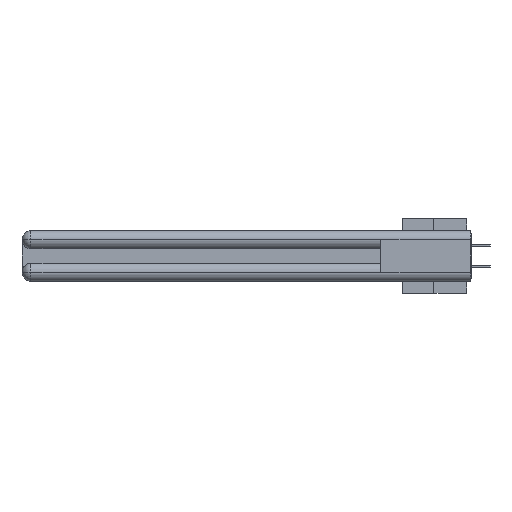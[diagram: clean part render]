
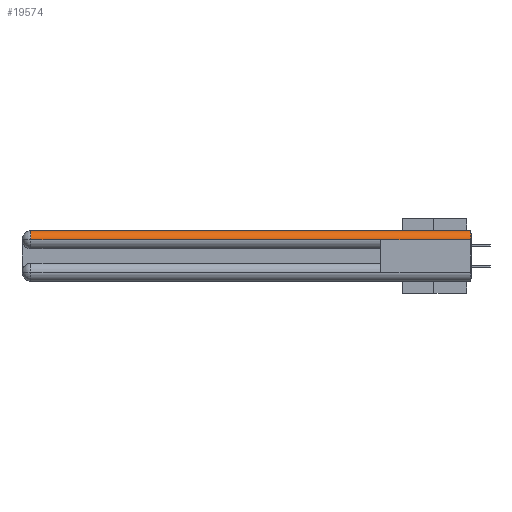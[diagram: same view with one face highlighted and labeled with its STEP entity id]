
A CAD part, left-side view. The second image highlights one B-rep face of the part: STEP entity #19574.
In plain terms, the highlighted cylindrical face has radius 1.562 mm (diameter 3.124 mm), a partial arc.
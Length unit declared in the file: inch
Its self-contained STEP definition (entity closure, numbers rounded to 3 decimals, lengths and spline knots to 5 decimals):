
#745 = CARTESIAN_POINT ( 'NONE',  ( 0.0615, 0., 0. ) ) ;
#1488 = LINE ( 'NONE', #22028, #15301 ) ;
#3059 = ORIENTED_EDGE ( 'NONE', *, *, #26582, .F. ) ;
#3536 = EDGE_CURVE ( 'NONE', #7636, #10527, #1488, .T. ) ;
#4419 = CARTESIAN_POINT ( 'NONE',  ( 0., 0., -0.0615 ) ) ;
#4798 = DIRECTION ( 'NONE',  ( 0., 0., 1. ) ) ;
#6450 = CARTESIAN_POINT ( 'NONE',  ( 0.0615, 0., -0.0615 ) ) ;
#6744 = DIRECTION ( 'NONE',  ( 0., -1., 0. ) ) ;
#7076 = ORIENTED_EDGE ( 'NONE', *, *, #29067, .T. ) ;
#7636 = VERTEX_POINT ( 'NONE', #24703 ) ;
#8125 = DIRECTION ( 'NONE',  ( 0., 1., 0. ) ) ;
#8323 = DIRECTION ( 'NONE',  ( 0., -1., 0. ) ) ;
#8765 = CARTESIAN_POINT ( 'NONE',  ( 0.0615, 2.94, 0. ) ) ;
#10527 = VERTEX_POINT ( 'NONE', #36685 ) ;
#11017 = FACE_OUTER_BOUND ( 'NONE', #36769, .T. ) ;
#11836 = CARTESIAN_POINT ( 'NONE',  ( 0.0615, 0., -0.0615 ) ) ;
#12681 = AXIS2_PLACEMENT_3D ( 'NONE', #6450, #6744, #23587 ) ;
#15301 = VECTOR ( 'NONE', #8323, 39.37008 ) ;
#17006 = CIRCLE ( 'NONE', #12681, 0.0615 ) ;
#17714 = VECTOR ( 'NONE', #24565, 39.37008 ) ;
#19574 = ADVANCED_FACE ( 'NONE', ( #11017 ), #34522, .T. ) ;
#20646 = VERTEX_POINT ( 'NONE', #40962 ) ;
#21542 = ORIENTED_EDGE ( 'NONE', *, *, #36132, .F. ) ;
#21773 = DIRECTION ( 'NONE',  ( 0., -1., 0. ) ) ;
#21914 = CARTESIAN_POINT ( 'NONE',  ( 0.0615, 2.94, -0.0615 ) ) ;
#22028 = CARTESIAN_POINT ( 'NONE',  ( 0., 3., -0.0615 ) ) ;
#22873 = CARTESIAN_POINT ( 'NONE',  ( 0., 3., -0.0615 ) ) ;
#23587 = DIRECTION ( 'NONE',  ( 1., 0., 0. ) ) ;
#24190 = EDGE_CURVE ( 'NONE', #24482, #20646, #27334, .T. ) ;
#24482 = VERTEX_POINT ( 'NONE', #8765 ) ;
#24512 = LINE ( 'NONE', #22873, #38983 ) ;
#24565 = DIRECTION ( 'NONE',  ( 0., -1., 0. ) ) ;
#24703 = CARTESIAN_POINT ( 'NONE',  ( 0., 2.94, -0.0615 ) ) ;
#25871 = DIRECTION ( 'NONE',  ( 0., 0., 1. ) ) ;
#25942 = AXIS2_PLACEMENT_3D ( 'NONE', #21914, #21773, #4798 ) ;
#26307 = DIRECTION ( 'NONE',  ( 0., 1., 0. ) ) ;
#26582 = EDGE_CURVE ( 'NONE', #40825, #10527, #24512, .T. ) ;
#27334 = LINE ( 'NONE', #745, #17714 ) ;
#27359 = ORIENTED_EDGE ( 'NONE', *, *, #24190, .F. ) ;
#29067 = EDGE_CURVE ( 'NONE', #24482, #7636, #33386, .T. ) ;
#29467 = AXIS2_PLACEMENT_3D ( 'NONE', #11836, #8125, #25871 ) ;
#31067 = ORIENTED_EDGE ( 'NONE', *, *, #3536, .T. ) ;
#33386 = CIRCLE ( 'NONE', #25942, 0.0615 ) ;
#34522 = CYLINDRICAL_SURFACE ( 'NONE', #29467, 0.0615 ) ;
#36132 = EDGE_CURVE ( 'NONE', #20646, #40825, #17006, .T. ) ;
#36685 = CARTESIAN_POINT ( 'NONE',  ( 0., 0.6, -0.0615 ) ) ;
#36769 = EDGE_LOOP ( 'NONE', ( #27359, #7076, #31067, #3059, #21542 ) ) ;
#38983 = VECTOR ( 'NONE', #26307, 39.37008 ) ;
#40825 = VERTEX_POINT ( 'NONE', #4419 ) ;
#40962 = CARTESIAN_POINT ( 'NONE',  ( 0.0615, 0., 0. ) ) ;
